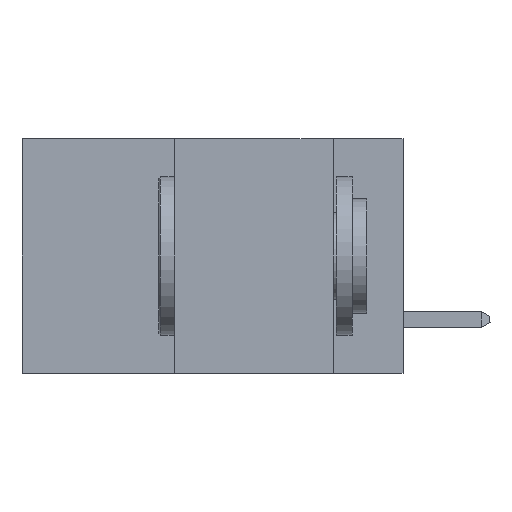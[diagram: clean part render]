
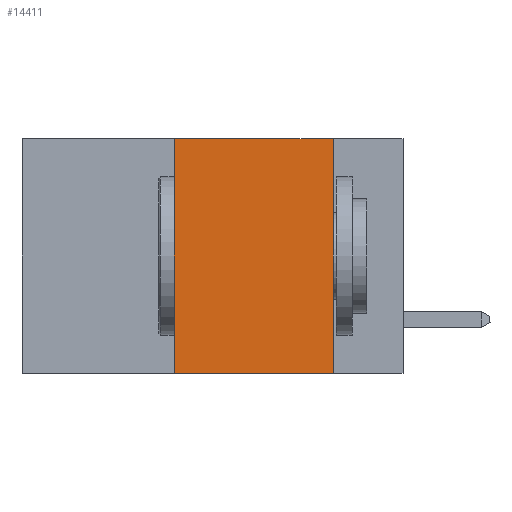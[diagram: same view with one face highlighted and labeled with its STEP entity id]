
A CAD part, left-side view. The second image highlights one B-rep face of the part: STEP entity #14411.
In plain terms, the highlighted planar face has unit normal (-1, 0, 0).
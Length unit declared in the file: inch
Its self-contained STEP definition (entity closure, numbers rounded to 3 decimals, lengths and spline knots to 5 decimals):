
#476 = LINE ( 'NONE', #13659, #9305 ) ;
#1451 = CARTESIAN_POINT ( 'NONE',  ( 0., 0.36, 0. ) ) ;
#2494 = AXIS2_PLACEMENT_3D ( 'NONE', #8004, #14660, #4767 ) ;
#3116 = PLANE ( 'NONE',  #2494 ) ;
#3427 = VERTEX_POINT ( 'NONE', #6995 ) ;
#3482 = VECTOR ( 'NONE', #4665, 39.37008 ) ;
#4665 = DIRECTION ( 'NONE',  ( 0., -1., 0. ) ) ;
#4767 = DIRECTION ( 'NONE',  ( 0., 0., -1. ) ) ;
#6620 = EDGE_CURVE ( 'NONE', #3427, #19205, #8143, .T. ) ;
#6995 = CARTESIAN_POINT ( 'NONE',  ( 0., 0.11, 0. ) ) ;
#7892 = CARTESIAN_POINT ( 'NONE',  ( 0., 0.11, -0.37 ) ) ;
#7914 = ORIENTED_EDGE ( 'NONE', *, *, #6620, .F. ) ;
#8004 = CARTESIAN_POINT ( 'NONE',  ( 0., 0.6, 0. ) ) ;
#8143 = LINE ( 'NONE', #12356, #20669 ) ;
#8929 = VECTOR ( 'NONE', #11451, 39.37008 ) ;
#9305 = VECTOR ( 'NONE', #10270, 39.37008 ) ;
#10270 = DIRECTION ( 'NONE',  ( 0., -1., 0. ) ) ;
#11451 = DIRECTION ( 'NONE',  ( 0., 0., 1. ) ) ;
#11655 = VERTEX_POINT ( 'NONE', #15676 ) ;
#12356 = CARTESIAN_POINT ( 'NONE',  ( 0., 0.11, 0. ) ) ;
#12850 = ORIENTED_EDGE ( 'NONE', *, *, #16998, .F. ) ;
#13625 = EDGE_LOOP ( 'NONE', ( #7914, #12850, #17182, #17698 ) ) ;
#13659 = CARTESIAN_POINT ( 'NONE',  ( 0., 0.6, -0.37 ) ) ;
#13661 = EDGE_CURVE ( 'NONE', #11655, #14978, #14865, .T. ) ;
#13907 = DIRECTION ( 'NONE',  ( 0., 0., -1. ) ) ;
#14411 = ADVANCED_FACE ( 'NONE', ( #15846 ), #3116, .F. ) ;
#14660 = DIRECTION ( 'NONE',  ( 1., 0., 0. ) ) ;
#14865 = LINE ( 'NONE', #1451, #8929 ) ;
#14978 = VERTEX_POINT ( 'NONE', #20924 ) ;
#15676 = CARTESIAN_POINT ( 'NONE',  ( 0., 0.36, -0.37 ) ) ;
#15846 = FACE_OUTER_BOUND ( 'NONE', #13625, .T. ) ;
#16998 = EDGE_CURVE ( 'NONE', #14978, #3427, #20897, .T. ) ;
#17182 = ORIENTED_EDGE ( 'NONE', *, *, #13661, .F. ) ;
#17698 = ORIENTED_EDGE ( 'NONE', *, *, #19510, .T. ) ;
#19205 = VERTEX_POINT ( 'NONE', #7892 ) ;
#19510 = EDGE_CURVE ( 'NONE', #11655, #19205, #476, .T. ) ;
#20669 = VECTOR ( 'NONE', #13907, 39.37008 ) ;
#20897 = LINE ( 'NONE', #20983, #3482 ) ;
#20924 = CARTESIAN_POINT ( 'NONE',  ( 0., 0.36, 0. ) ) ;
#20983 = CARTESIAN_POINT ( 'NONE',  ( 0., 0.6, 0. ) ) ;
